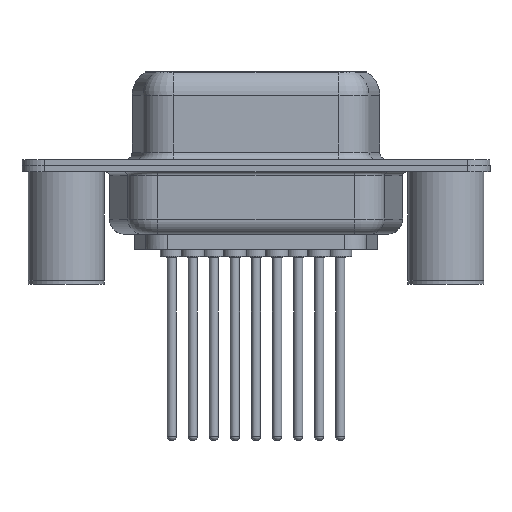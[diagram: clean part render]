
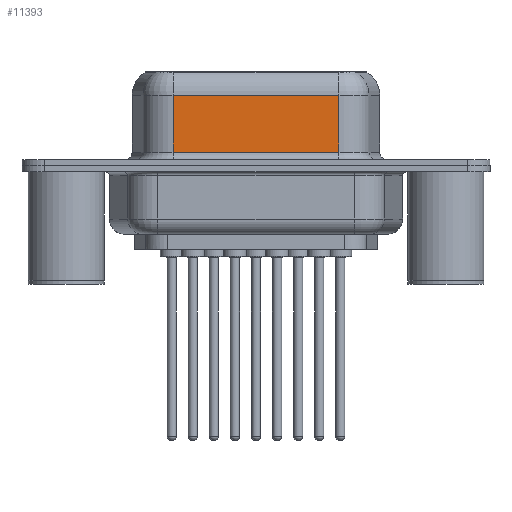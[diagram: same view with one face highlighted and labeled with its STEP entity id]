
A CAD part, front view. The second image highlights one B-rep face of the part: STEP entity #11393.
In plain terms, the highlighted planar face has unit normal (0, -1, 0).
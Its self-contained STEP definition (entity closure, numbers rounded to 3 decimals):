
#480 = CARTESIAN_POINT ( 'NONE',  ( 17.962, -3.95, 0.9 ) ) ;
#735 = DIRECTION ( 'NONE',  ( 0., 0., -1. ) ) ;
#773 = PLANE ( 'NONE',  #4939 ) ;
#915 = VECTOR ( 'NONE', #6893, 1000. ) ;
#1407 = VERTEX_POINT ( 'NONE', #10010 ) ;
#1426 = VECTOR ( 'NONE', #735, 1000. ) ;
#1806 = CARTESIAN_POINT ( 'NONE',  ( 7.038, -3.95, 6.4 ) ) ;
#2475 = ORIENTED_EDGE ( 'NONE', *, *, #6520, .T. ) ;
#2822 = CARTESIAN_POINT ( 'NONE',  ( 7.038, -3.95, 0.9 ) ) ;
#4552 = ORIENTED_EDGE ( 'NONE', *, *, #12890, .T. ) ;
#4939 = AXIS2_PLACEMENT_3D ( 'NONE', #8223, #5780, #15561 ) ;
#5428 = LINE ( 'NONE', #1806, #915 ) ;
#5780 = DIRECTION ( 'NONE',  ( 0., 1., 0. ) ) ;
#6059 = EDGE_CURVE ( 'NONE', #14134, #1407, #7950, .T. ) ;
#6520 = EDGE_CURVE ( 'NONE', #7330, #1407, #9167, .T. ) ;
#6706 = DIRECTION ( 'NONE',  ( 1., 0., 0. ) ) ;
#6893 = DIRECTION ( 'NONE',  ( 0., 0., -1. ) ) ;
#7101 = CARTESIAN_POINT ( 'NONE',  ( 17.962, -3.95, 4.65 ) ) ;
#7330 = VERTEX_POINT ( 'NONE', #2822 ) ;
#7717 = ORIENTED_EDGE ( 'NONE', *, *, #6059, .F. ) ;
#7950 = LINE ( 'NONE', #11922, #1426 ) ;
#8223 = CARTESIAN_POINT ( 'NONE',  ( 17.962, -3.95, 6.4 ) ) ;
#8310 = FACE_OUTER_BOUND ( 'NONE', #16018, .T. ) ;
#8989 = CARTESIAN_POINT ( 'NONE',  ( 7.038, -3.95, 4.65 ) ) ;
#9167 = LINE ( 'NONE', #480, #15786 ) ;
#9300 = CARTESIAN_POINT ( 'NONE',  ( 17.962, -3.95, 4.65 ) ) ;
#10010 = CARTESIAN_POINT ( 'NONE',  ( 17.962, -3.95, 0.9 ) ) ;
#11393 = ADVANCED_FACE ( 'NONE', ( #8310 ), #773, .F. ) ;
#11922 = CARTESIAN_POINT ( 'NONE',  ( 17.962, -3.95, 6.4 ) ) ;
#12045 = DIRECTION ( 'NONE',  ( -1., 0., 0. ) ) ;
#12371 = VECTOR ( 'NONE', #12045, 1000. ) ;
#12890 = EDGE_CURVE ( 'NONE', #14134, #14038, #13593, .T. ) ;
#13593 = LINE ( 'NONE', #7101, #12371 ) ;
#13663 = EDGE_CURVE ( 'NONE', #14038, #7330, #5428, .T. ) ;
#14038 = VERTEX_POINT ( 'NONE', #8989 ) ;
#14134 = VERTEX_POINT ( 'NONE', #9300 ) ;
#14248 = ORIENTED_EDGE ( 'NONE', *, *, #13663, .T. ) ;
#15561 = DIRECTION ( 'NONE',  ( 0., 0., 1. ) ) ;
#15786 = VECTOR ( 'NONE', #6706, 1000. ) ;
#16018 = EDGE_LOOP ( 'NONE', ( #7717, #4552, #14248, #2475 ) ) ;
